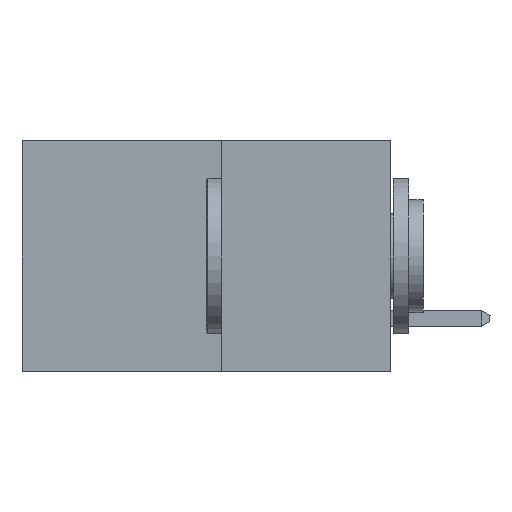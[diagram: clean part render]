
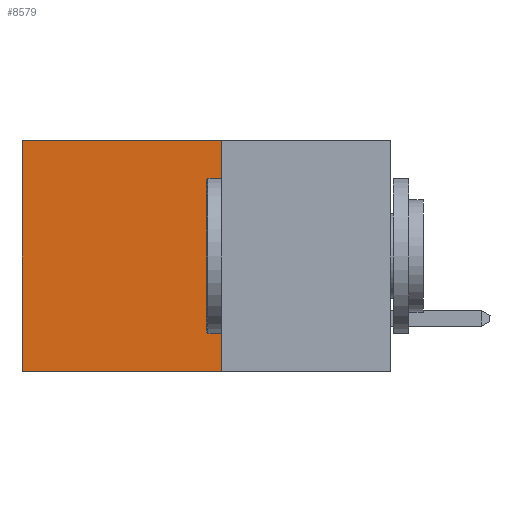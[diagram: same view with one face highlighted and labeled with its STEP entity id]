
A CAD part, left-side view. The second image highlights one B-rep face of the part: STEP entity #8579.
In plain terms, the highlighted planar face has unit normal (-1, 0, 0).
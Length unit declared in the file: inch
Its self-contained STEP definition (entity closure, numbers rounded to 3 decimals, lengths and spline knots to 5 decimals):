
#1423 = DIRECTION ( 'NONE',  ( 0., 0., -1. ) ) ;
#1443 = CARTESIAN_POINT ( 'NONE',  ( 0.277, 0.27, 0. ) ) ;
#1992 = VECTOR ( 'NONE', #13077, 39.37008 ) ;
#2576 = VERTEX_POINT ( 'NONE', #18584 ) ;
#2995 = LINE ( 'NONE', #5642, #9346 ) ;
#3029 = VECTOR ( 'NONE', #15805, 39.37008 ) ;
#3080 = VERTEX_POINT ( 'NONE', #8263 ) ;
#3211 = EDGE_CURVE ( 'NONE', #3080, #4071, #22168, .T. ) ;
#3965 = AXIS2_PLACEMENT_3D ( 'NONE', #7694, #10107, #26889 ) ;
#4071 = VERTEX_POINT ( 'NONE', #14520 ) ;
#4789 = EDGE_CURVE ( 'NONE', #3080, #2576, #27494, .T. ) ;
#5167 = VECTOR ( 'NONE', #1423, 39.37008 ) ;
#5642 = CARTESIAN_POINT ( 'NONE',  ( 0.277, 0.27, -0.37 ) ) ;
#7694 = CARTESIAN_POINT ( 'NONE',  ( 0.277, 0.27, -0.37 ) ) ;
#8043 = DIRECTION ( 'NONE',  ( 0., 1., 0. ) ) ;
#8263 = CARTESIAN_POINT ( 'NONE',  ( 0.277, 0.27, 0. ) ) ;
#8579 = ADVANCED_FACE ( 'NONE', ( #15234 ), #22070, .F. ) ;
#9346 = VECTOR ( 'NONE', #8043, 39.37008 ) ;
#10107 = DIRECTION ( 'NONE',  ( 1., 0., 0. ) ) ;
#11253 = ORIENTED_EDGE ( 'NONE', *, *, #30501, .F. ) ;
#12180 = EDGE_LOOP ( 'NONE', ( #13444, #11253, #24160, #14712 ) ) ;
#13077 = DIRECTION ( 'NONE',  ( 0., 0., -1. ) ) ;
#13385 = EDGE_CURVE ( 'NONE', #4071, #16819, #22797, .T. ) ;
#13444 = ORIENTED_EDGE ( 'NONE', *, *, #13385, .T. ) ;
#14066 = CARTESIAN_POINT ( 'NONE',  ( 0.277, 0.59, -0.37 ) ) ;
#14520 = CARTESIAN_POINT ( 'NONE',  ( 0.277, 0.59, 0. ) ) ;
#14712 = ORIENTED_EDGE ( 'NONE', *, *, #3211, .T. ) ;
#15234 = FACE_OUTER_BOUND ( 'NONE', #12180, .T. ) ;
#15805 = DIRECTION ( 'NONE',  ( 0., 1., 0. ) ) ;
#16819 = VERTEX_POINT ( 'NONE', #14066 ) ;
#17911 = CARTESIAN_POINT ( 'NONE',  ( 0.277, 0.27, -0.37 ) ) ;
#18584 = CARTESIAN_POINT ( 'NONE',  ( 0.277, 0.27, -0.37 ) ) ;
#22070 = PLANE ( 'NONE',  #3965 ) ;
#22168 = LINE ( 'NONE', #1443, #3029 ) ;
#22797 = LINE ( 'NONE', #30121, #5167 ) ;
#24160 = ORIENTED_EDGE ( 'NONE', *, *, #4789, .F. ) ;
#26889 = DIRECTION ( 'NONE',  ( 0., 0., -1. ) ) ;
#27494 = LINE ( 'NONE', #17911, #1992 ) ;
#30121 = CARTESIAN_POINT ( 'NONE',  ( 0.277, 0.59, -0.37 ) ) ;
#30501 = EDGE_CURVE ( 'NONE', #2576, #16819, #2995, .T. ) ;
